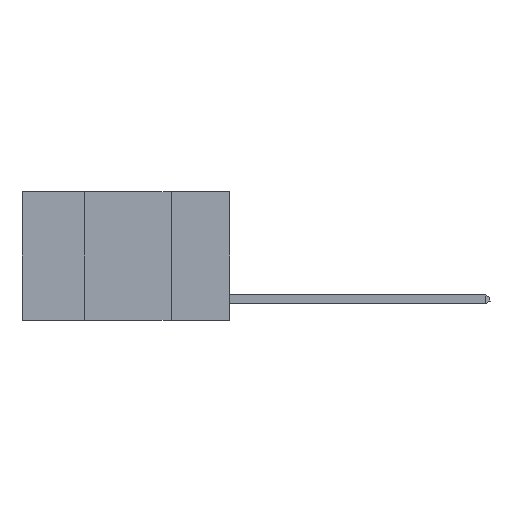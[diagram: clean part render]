
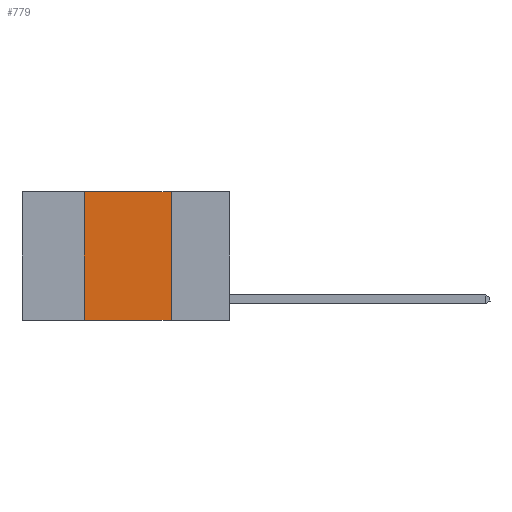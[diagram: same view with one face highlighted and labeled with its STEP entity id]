
A CAD part, left-side view. The second image highlights one B-rep face of the part: STEP entity #779.
In plain terms, the highlighted planar face has unit normal (-1, 0, 0).
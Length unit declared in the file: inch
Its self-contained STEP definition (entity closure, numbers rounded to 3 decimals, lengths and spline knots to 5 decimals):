
#669 = FACE_OUTER_BOUND ( 'NONE', #7634, .T. ) ;
#779 = ADVANCED_FACE ( 'NONE', ( #669 ), #7589, .F. ) ;
#1555 = CARTESIAN_POINT ( 'NONE',  ( 0., 0.17, 0. ) ) ;
#1969 = EDGE_CURVE ( 'NONE', #6937, #10545, #10325, .T. ) ;
#2609 = CARTESIAN_POINT ( 'NONE',  ( 0., 0.6, 0. ) ) ;
#2973 = ORIENTED_EDGE ( 'NONE', *, *, #3779, .F. ) ;
#2994 = CARTESIAN_POINT ( 'NONE',  ( 0., 0.42, 0. ) ) ;
#3237 = LINE ( 'NONE', #11494, #7869 ) ;
#3779 = EDGE_CURVE ( 'NONE', #12762, #12185, #8879, .T. ) ;
#4248 = ORIENTED_EDGE ( 'NONE', *, *, #7105, .F. ) ;
#4554 = VECTOR ( 'NONE', #8652, 39.37008 ) ;
#4791 = CARTESIAN_POINT ( 'NONE',  ( 0., 0.42, -0.37 ) ) ;
#5424 = VECTOR ( 'NONE', #5447, 39.37008 ) ;
#5447 = DIRECTION ( 'NONE',  ( 0., -1., 0. ) ) ;
#5718 = DIRECTION ( 'NONE',  ( 0., 0., -1. ) ) ;
#6349 = EDGE_CURVE ( 'NONE', #6937, #12185, #3237, .T. ) ;
#6790 = CARTESIAN_POINT ( 'NONE',  ( 0., 0.17, -0.37 ) ) ;
#6937 = VERTEX_POINT ( 'NONE', #4791 ) ;
#7075 = CARTESIAN_POINT ( 'NONE',  ( 0., 0.17, 0. ) ) ;
#7105 = EDGE_CURVE ( 'NONE', #10545, #12762, #9274, .T. ) ;
#7589 = PLANE ( 'NONE',  #10837 ) ;
#7634 = EDGE_LOOP ( 'NONE', ( #2973, #4248, #9615, #9539 ) ) ;
#7869 = VECTOR ( 'NONE', #8523, 39.37008 ) ;
#8220 = DIRECTION ( 'NONE',  ( 0., 0., 1. ) ) ;
#8523 = DIRECTION ( 'NONE',  ( 0., -1., 0. ) ) ;
#8652 = DIRECTION ( 'NONE',  ( 0., 0., -1. ) ) ;
#8879 = LINE ( 'NONE', #1555, #4554 ) ;
#9274 = LINE ( 'NONE', #10684, #5424 ) ;
#9539 = ORIENTED_EDGE ( 'NONE', *, *, #6349, .T. ) ;
#9615 = ORIENTED_EDGE ( 'NONE', *, *, #1969, .F. ) ;
#10325 = LINE ( 'NONE', #12188, #12813 ) ;
#10545 = VERTEX_POINT ( 'NONE', #2994 ) ;
#10684 = CARTESIAN_POINT ( 'NONE',  ( 0., 0.6, 0. ) ) ;
#10837 = AXIS2_PLACEMENT_3D ( 'NONE', #2609, #11795, #5718 ) ;
#11494 = CARTESIAN_POINT ( 'NONE',  ( 0., 0.6, -0.37 ) ) ;
#11795 = DIRECTION ( 'NONE',  ( 1., 0., 0. ) ) ;
#12185 = VERTEX_POINT ( 'NONE', #6790 ) ;
#12188 = CARTESIAN_POINT ( 'NONE',  ( 0., 0.42, 0. ) ) ;
#12762 = VERTEX_POINT ( 'NONE', #7075 ) ;
#12813 = VECTOR ( 'NONE', #8220, 39.37008 ) ;
